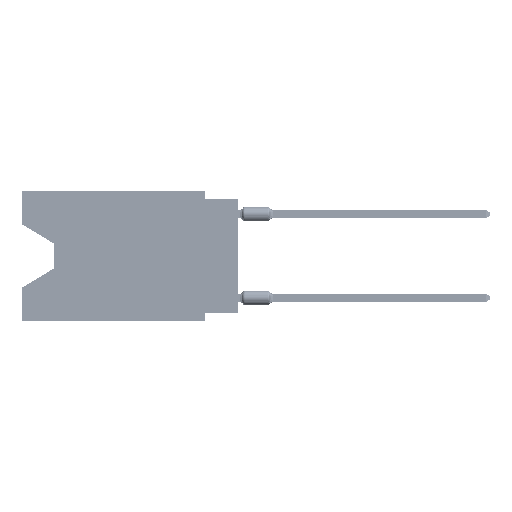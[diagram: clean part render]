
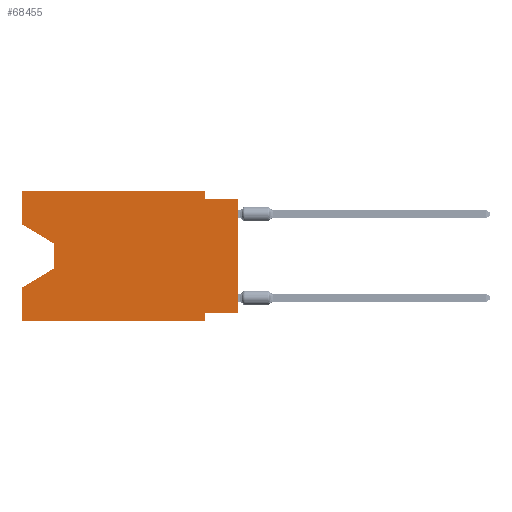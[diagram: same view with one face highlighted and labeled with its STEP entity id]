
A CAD part, left-side view. The second image highlights one B-rep face of the part: STEP entity #68455.
In plain terms, the highlighted planar face has unit normal (-1, 0, 0).
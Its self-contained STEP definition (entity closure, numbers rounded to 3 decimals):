
#964 = LINE ( 'NONE', #41385, #9454 ) ;
#1907 = LINE ( 'NONE', #41555, #19421 ) ;
#2287 = DIRECTION ( 'NONE',  ( 0., -0.855, -0.519 ) ) ;
#3054 = LINE ( 'NONE', #25359, #31848 ) ;
#3544 = VERTEX_POINT ( 'NONE', #49672 ) ;
#4289 = ORIENTED_EDGE ( 'NONE', *, *, #13659, .T. ) ;
#5621 = CARTESIAN_POINT ( 'NONE',  ( 0., 16.383, 0. ) ) ;
#6614 = VECTOR ( 'NONE', #53837, 1000. ) ;
#8727 = VERTEX_POINT ( 'NONE', #21715 ) ;
#9454 = VECTOR ( 'NONE', #12688, 1000. ) ;
#9966 = EDGE_CURVE ( 'NONE', #8727, #40563, #33671, .T. ) ;
#10244 = DIRECTION ( 'NONE',  ( 0., 0.855, -0.519 ) ) ;
#10407 = ORIENTED_EDGE ( 'NONE', *, *, #36693, .T. ) ;
#10761 = EDGE_CURVE ( 'NONE', #3544, #40563, #23202, .T. ) ;
#11298 = DIRECTION ( 'NONE',  ( 0., 0., -1. ) ) ;
#11490 = DIRECTION ( 'NONE',  ( 0., -1., 0. ) ) ;
#11668 = FACE_OUTER_BOUND ( 'NONE', #62386, .T. ) ;
#11972 = ORIENTED_EDGE ( 'NONE', *, *, #21152, .F. ) ;
#12017 = CARTESIAN_POINT ( 'NONE',  ( 0., 2.54, -0.635 ) ) ;
#12468 = ORIENTED_EDGE ( 'NONE', *, *, #68408, .T. ) ;
#12688 = DIRECTION ( 'NONE',  ( 0., -1., 0. ) ) ;
#12927 = DIRECTION ( 'NONE',  ( 0., 0., 1. ) ) ;
#13659 = EDGE_CURVE ( 'NONE', #14226, #24144, #68396, .T. ) ;
#13836 = LINE ( 'NONE', #70873, #19355 ) ;
#14226 = VERTEX_POINT ( 'NONE', #33198 ) ;
#15643 = CARTESIAN_POINT ( 'NONE',  ( 0., 16.383, 0. ) ) ;
#16759 = DIRECTION ( 'NONE',  ( 0., 0., 1. ) ) ;
#16949 = DIRECTION ( 'NONE',  ( 0., 0., -1. ) ) ;
#17484 = VECTOR ( 'NONE', #10244, 1000. ) ;
#17626 = EDGE_CURVE ( 'NONE', #27740, #73272, #964, .T. ) ;
#17740 = EDGE_CURVE ( 'NONE', #3544, #24144, #68503, .T. ) ;
#19355 = VECTOR ( 'NONE', #47073, 1000. ) ;
#19421 = VECTOR ( 'NONE', #2287, 1000. ) ;
#20071 = EDGE_CURVE ( 'NONE', #30808, #30382, #13836, .T. ) ;
#20112 = CARTESIAN_POINT ( 'NONE',  ( 0., 16.383, -7.36 ) ) ;
#21152 = EDGE_CURVE ( 'NONE', #24601, #27740, #24264, .T. ) ;
#21715 = CARTESIAN_POINT ( 'NONE',  ( 0., 2.54, -9.271 ) ) ;
#21933 = CARTESIAN_POINT ( 'NONE',  ( 0., 0., -9.271 ) ) ;
#22244 = CARTESIAN_POINT ( 'NONE',  ( 0., 13.97, -4.013 ) ) ;
#23158 = CARTESIAN_POINT ( 'NONE',  ( 0., 16.383, 0. ) ) ;
#23202 = LINE ( 'NONE', #57934, #72484 ) ;
#24144 = VERTEX_POINT ( 'NONE', #20112 ) ;
#24264 = LINE ( 'NONE', #23158, #47221 ) ;
#24601 = VERTEX_POINT ( 'NONE', #58943 ) ;
#25359 = CARTESIAN_POINT ( 'NONE',  ( 0., 0., 0. ) ) ;
#25893 = EDGE_CURVE ( 'NONE', #73272, #30808, #46001, .T. ) ;
#26220 = CARTESIAN_POINT ( 'NONE',  ( 0., 2.54, -9.906 ) ) ;
#26448 = EDGE_CURVE ( 'NONE', #39940, #8727, #36453, .T. ) ;
#27740 = VERTEX_POINT ( 'NONE', #15643 ) ;
#28786 = VECTOR ( 'NONE', #16949, 1000. ) ;
#29449 = CARTESIAN_POINT ( 'NONE',  ( 0., 0., -0.635 ) ) ;
#30181 = ORIENTED_EDGE ( 'NONE', *, *, #20071, .F. ) ;
#30206 = VECTOR ( 'NONE', #62004, 1000. ) ;
#30382 = VERTEX_POINT ( 'NONE', #29449 ) ;
#30808 = VERTEX_POINT ( 'NONE', #12017 ) ;
#31848 = VECTOR ( 'NONE', #66521, 1000. ) ;
#32297 = CARTESIAN_POINT ( 'NONE',  ( 0., 2.54, 0. ) ) ;
#33198 = CARTESIAN_POINT ( 'NONE',  ( 0., 13.97, -5.893 ) ) ;
#33671 = LINE ( 'NONE', #40081, #30206 ) ;
#36453 = LINE ( 'NONE', #71190, #6614 ) ;
#36693 = EDGE_CURVE ( 'NONE', #24601, #60199, #1907, .T. ) ;
#37207 = VECTOR ( 'NONE', #16759, 1000. ) ;
#38448 = AXIS2_PLACEMENT_3D ( 'NONE', #5621, #45267, #11298 ) ;
#38937 = CARTESIAN_POINT ( 'NONE',  ( 0., 13.97, -5.893 ) ) ;
#39548 = ORIENTED_EDGE ( 'NONE', *, *, #25893, .F. ) ;
#39940 = VERTEX_POINT ( 'NONE', #21933 ) ;
#40081 = CARTESIAN_POINT ( 'NONE',  ( 0., 2.54, -9.906 ) ) ;
#40563 = VERTEX_POINT ( 'NONE', #26220 ) ;
#41385 = CARTESIAN_POINT ( 'NONE',  ( 0., 16.383, 0. ) ) ;
#41555 = CARTESIAN_POINT ( 'NONE',  ( 0., 16.383, -2.546 ) ) ;
#43465 = CARTESIAN_POINT ( 'NONE',  ( 0., 13.97, -4.013 ) ) ;
#45267 = DIRECTION ( 'NONE',  ( 1., 0., 0. ) ) ;
#45466 = CARTESIAN_POINT ( 'NONE',  ( 0., 16.383, 0. ) ) ;
#46001 = LINE ( 'NONE', #46362, #54838 ) ;
#46362 = CARTESIAN_POINT ( 'NONE',  ( 0., 2.54, 0. ) ) ;
#47073 = DIRECTION ( 'NONE',  ( 0., -1., 0. ) ) ;
#47221 = VECTOR ( 'NONE', #12927, 1000. ) ;
#49672 = CARTESIAN_POINT ( 'NONE',  ( 0., 16.383, -9.906 ) ) ;
#52850 = ORIENTED_EDGE ( 'NONE', *, *, #9966, .F. ) ;
#53837 = DIRECTION ( 'NONE',  ( 0., 1., 0. ) ) ;
#54838 = VECTOR ( 'NONE', #57699, 1000. ) ;
#54993 = ORIENTED_EDGE ( 'NONE', *, *, #17740, .F. ) ;
#57355 = LINE ( 'NONE', #22244, #28786 ) ;
#57699 = DIRECTION ( 'NONE',  ( 0., 0., -1. ) ) ;
#57934 = CARTESIAN_POINT ( 'NONE',  ( 0., 16.383, -9.906 ) ) ;
#58943 = CARTESIAN_POINT ( 'NONE',  ( 0., 16.383, -2.546 ) ) ;
#58984 = EDGE_CURVE ( 'NONE', #39940, #30382, #3054, .T. ) ;
#60199 = VERTEX_POINT ( 'NONE', #43465 ) ;
#60957 = ORIENTED_EDGE ( 'NONE', *, *, #58984, .T. ) ;
#62004 = DIRECTION ( 'NONE',  ( 0., 0., -1. ) ) ;
#62386 = EDGE_LOOP ( 'NONE', ( #10407, #12468, #4289, #54993, #65034, #52850, #70018, #60957, #30181, #39548, #72233, #11972 ) ) ;
#63030 = PLANE ( 'NONE',  #38448 ) ;
#65034 = ORIENTED_EDGE ( 'NONE', *, *, #10761, .T. ) ;
#66521 = DIRECTION ( 'NONE',  ( 0., 0., 1. ) ) ;
#68396 = LINE ( 'NONE', #38937, #17484 ) ;
#68408 = EDGE_CURVE ( 'NONE', #60199, #14226, #57355, .T. ) ;
#68455 = ADVANCED_FACE ( 'NONE', ( #11668 ), #63030, .F. ) ;
#68503 = LINE ( 'NONE', #45466, #37207 ) ;
#70018 = ORIENTED_EDGE ( 'NONE', *, *, #26448, .F. ) ;
#70873 = CARTESIAN_POINT ( 'NONE',  ( 0., 0., -0.635 ) ) ;
#71190 = CARTESIAN_POINT ( 'NONE',  ( 0., 0., -9.271 ) ) ;
#72233 = ORIENTED_EDGE ( 'NONE', *, *, #17626, .F. ) ;
#72484 = VECTOR ( 'NONE', #11490, 1000. ) ;
#73272 = VERTEX_POINT ( 'NONE', #32297 ) ;
